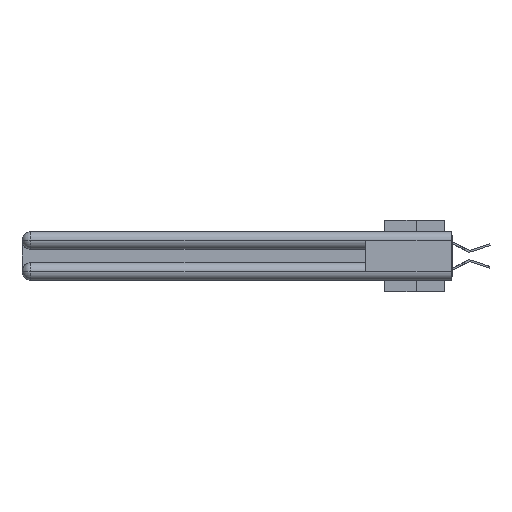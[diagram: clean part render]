
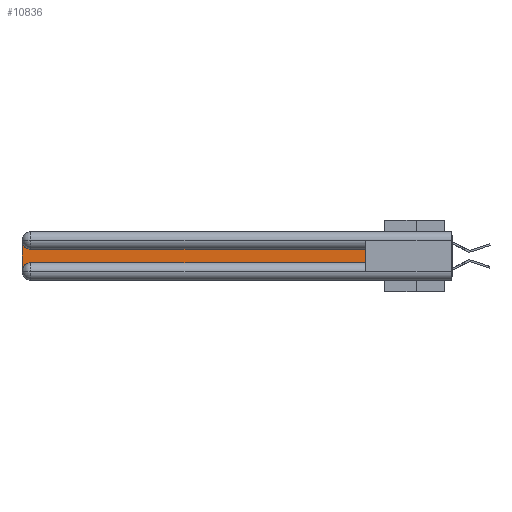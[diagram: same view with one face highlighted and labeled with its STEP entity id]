
A CAD part, left-side view. The second image highlights one B-rep face of the part: STEP entity #10836.
In plain terms, the highlighted planar face has unit normal (-1, 0, 0).
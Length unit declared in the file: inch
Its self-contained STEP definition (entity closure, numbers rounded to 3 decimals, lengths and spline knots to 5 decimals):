
#220 = DIRECTION ( 'NONE',  ( 1., 0., 0. ) ) ;
#690 = VERTEX_POINT ( 'NONE', #10242 ) ;
#755 = DIRECTION ( 'NONE',  ( 1., 0., 0. ) ) ;
#1030 = LINE ( 'NONE', #20855, #17709 ) ;
#1819 = EDGE_CURVE ( 'NONE', #18944, #5862, #9567, .T. ) ;
#2118 = CARTESIAN_POINT ( 'NONE',  ( 0.075, 0.6, -0.2175 ) ) ;
#2677 = CARTESIAN_POINT ( 'NONE',  ( 0.075, 2.94, -0.1225 ) ) ;
#2906 = EDGE_CURVE ( 'NONE', #14762, #18944, #1030, .T. ) ;
#3126 = CIRCLE ( 'NONE', #11962, 0.06 ) ;
#3770 = CIRCLE ( 'NONE', #14670, 0.06 ) ;
#4681 = EDGE_CURVE ( 'NONE', #16061, #14762, #11388, .T. ) ;
#5862 = VERTEX_POINT ( 'NONE', #2677 ) ;
#5905 = CARTESIAN_POINT ( 'NONE',  ( 0.075, 2.94, -0.2175 ) ) ;
#6152 = CARTESIAN_POINT ( 'NONE',  ( 0.075, 3., -0.2175 ) ) ;
#6499 = VECTOR ( 'NONE', #21469, 39.37008 ) ;
#7673 = CARTESIAN_POINT ( 'NONE',  ( 0.075, 0.6, -0.1225 ) ) ;
#9567 = LINE ( 'NONE', #19476, #29915 ) ;
#10242 = CARTESIAN_POINT ( 'NONE',  ( 0.075, 3., -0.2775 ) ) ;
#10836 = ADVANCED_FACE ( 'NONE', ( #23013 ), #21071, .F. ) ;
#11181 = ORIENTED_EDGE ( 'NONE', *, *, #1819, .T. ) ;
#11388 = LINE ( 'NONE', #2118, #6499 ) ;
#11603 = ORIENTED_EDGE ( 'NONE', *, *, #27560, .T. ) ;
#11962 = AXIS2_PLACEMENT_3D ( 'NONE', #25319, #27442, #14922 ) ;
#12165 = DIRECTION ( 'NONE',  ( 0., 1., 0. ) ) ;
#13049 = DIRECTION ( 'NONE',  ( 0., 0., 1. ) ) ;
#14670 = AXIS2_PLACEMENT_3D ( 'NONE', #30279, #220, #22334 ) ;
#14762 = VERTEX_POINT ( 'NONE', #30755 ) ;
#14922 = DIRECTION ( 'NONE',  ( 0., 0., -1. ) ) ;
#16061 = VERTEX_POINT ( 'NONE', #5905 ) ;
#17709 = VECTOR ( 'NONE', #13049, 39.37008 ) ;
#18599 = EDGE_CURVE ( 'NONE', #5862, #20660, #3770, .T. ) ;
#18944 = VERTEX_POINT ( 'NONE', #7673 ) ;
#19319 = ORIENTED_EDGE ( 'NONE', *, *, #4681, .T. ) ;
#19327 = ORIENTED_EDGE ( 'NONE', *, *, #18599, .T. ) ;
#19476 = CARTESIAN_POINT ( 'NONE',  ( 0.075, 0.6, -0.1225 ) ) ;
#20660 = VERTEX_POINT ( 'NONE', #28950 ) ;
#20855 = CARTESIAN_POINT ( 'NONE',  ( 0.075, 0.6, -0.2175 ) ) ;
#21071 = PLANE ( 'NONE',  #27850 ) ;
#21469 = DIRECTION ( 'NONE',  ( 0., -1., 0. ) ) ;
#22079 = ORIENTED_EDGE ( 'NONE', *, *, #23937, .T. ) ;
#22334 = DIRECTION ( 'NONE',  ( 0., 0., -1. ) ) ;
#23013 = FACE_OUTER_BOUND ( 'NONE', #27568, .T. ) ;
#23041 = LINE ( 'NONE', #6152, #29913 ) ;
#23937 = EDGE_CURVE ( 'NONE', #20660, #690, #23041, .T. ) ;
#25319 = CARTESIAN_POINT ( 'NONE',  ( 0.075, 2.94, -0.2775 ) ) ;
#26124 = DIRECTION ( 'NONE',  ( 0., 0., -1. ) ) ;
#27442 = DIRECTION ( 'NONE',  ( 1., 0., 0. ) ) ;
#27560 = EDGE_CURVE ( 'NONE', #690, #16061, #3126, .T. ) ;
#27568 = EDGE_LOOP ( 'NONE', ( #11181, #19327, #22079, #11603, #19319, #30194 ) ) ;
#27734 = CARTESIAN_POINT ( 'NONE',  ( 0.075, 3., -0.1225 ) ) ;
#27850 = AXIS2_PLACEMENT_3D ( 'NONE', #27734, #755, #30492 ) ;
#28950 = CARTESIAN_POINT ( 'NONE',  ( 0.075, 3., -0.0625 ) ) ;
#29913 = VECTOR ( 'NONE', #26124, 39.37008 ) ;
#29915 = VECTOR ( 'NONE', #12165, 39.37008 ) ;
#30194 = ORIENTED_EDGE ( 'NONE', *, *, #2906, .T. ) ;
#30279 = CARTESIAN_POINT ( 'NONE',  ( 0.075, 2.94, -0.0625 ) ) ;
#30492 = DIRECTION ( 'NONE',  ( 0., 0., -1. ) ) ;
#30755 = CARTESIAN_POINT ( 'NONE',  ( 0.075, 0.6, -0.2175 ) ) ;
